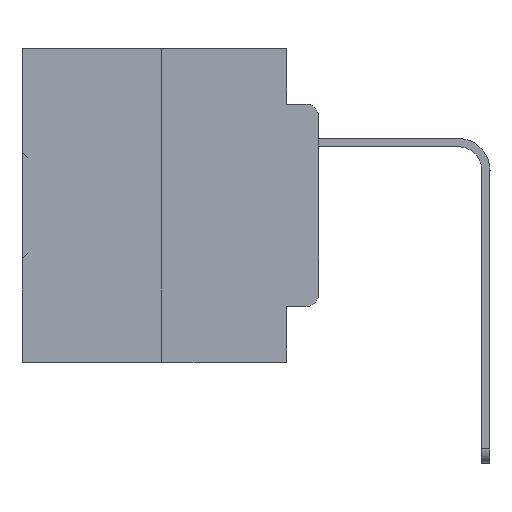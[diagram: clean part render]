
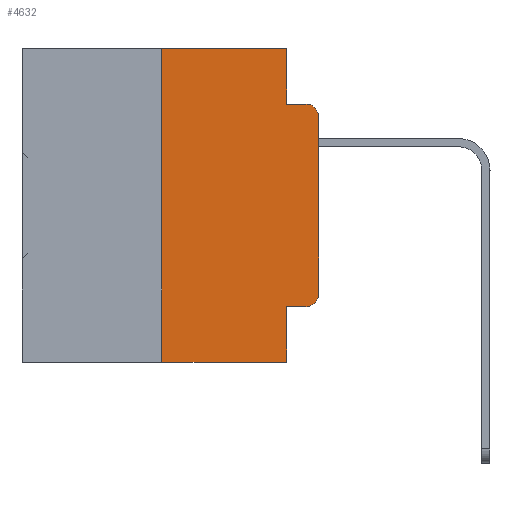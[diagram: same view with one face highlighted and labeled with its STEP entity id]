
A CAD part, left-side view. The second image highlights one B-rep face of the part: STEP entity #4632.
In plain terms, the highlighted planar face has unit normal (-1, 0, 0).
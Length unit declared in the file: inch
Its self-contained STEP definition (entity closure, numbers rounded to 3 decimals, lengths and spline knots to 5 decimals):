
#1252 = DIRECTION ( 'NONE',  ( 0., 0., -1. ) ) ;
#1343 = DIRECTION ( 'NONE',  ( 0., 0., -1. ) ) ;
#1459 = EDGE_CURVE ( 'NONE', #8099, #14613, #27639, .T. ) ;
#1803 = EDGE_CURVE ( 'NONE', #5049, #16139, #24611, .T. ) ;
#1824 = LINE ( 'NONE', #24914, #20456 ) ;
#1993 = LINE ( 'NONE', #28697, #35735 ) ;
#2382 = ORIENTED_EDGE ( 'NONE', *, *, #1803, .F. ) ;
#3555 = ORIENTED_EDGE ( 'NONE', *, *, #18162, .T. ) ;
#3873 = ORIENTED_EDGE ( 'NONE', *, *, #33376, .T. ) ;
#4410 = VERTEX_POINT ( 'NONE', #18798 ) ;
#4632 = ADVANCED_FACE ( 'NONE', ( #6417 ), #9212, .F. ) ;
#5018 = AXIS2_PLACEMENT_3D ( 'NONE', #8006, #21920, #16122 ) ;
#5049 = VERTEX_POINT ( 'NONE', #10887 ) ;
#5276 = CARTESIAN_POINT ( 'NONE',  ( 0., 0.473, -0.5 ) ) ;
#6052 = CARTESIAN_POINT ( 'NONE',  ( 0., 0.051, -0.5 ) ) ;
#6417 = FACE_OUTER_BOUND ( 'NONE', #10065, .T. ) ;
#6690 = ORIENTED_EDGE ( 'NONE', *, *, #1459, .T. ) ;
#7670 = ORIENTED_EDGE ( 'NONE', *, *, #20292, .F. ) ;
#8006 = CARTESIAN_POINT ( 'NONE',  ( 0., 0.02, -0.1085 ) ) ;
#8099 = VERTEX_POINT ( 'NONE', #27360 ) ;
#8934 = DIRECTION ( 'NONE',  ( 0., 0., -1. ) ) ;
#9212 = PLANE ( 'NONE',  #11813 ) ;
#9758 = ORIENTED_EDGE ( 'NONE', *, *, #31690, .F. ) ;
#10065 = EDGE_LOOP ( 'NONE', ( #6690, #16196, #12038, #7670, #9758, #2382, #22916, #22209, #3555, #3873 ) ) ;
#10873 = DIRECTION ( 'NONE',  ( 0., -1., 0. ) ) ;
#10887 = CARTESIAN_POINT ( 'NONE',  ( 0., 0.25, -0.5 ) ) ;
#10964 = CARTESIAN_POINT ( 'NONE',  ( 0., 0.051, 0. ) ) ;
#11242 = CARTESIAN_POINT ( 'NONE',  ( 0., 0.051, 0. ) ) ;
#11813 = AXIS2_PLACEMENT_3D ( 'NONE', #25563, #34114, #28425 ) ;
#12009 = VECTOR ( 'NONE', #32639, 39.37008 ) ;
#12038 = ORIENTED_EDGE ( 'NONE', *, *, #23349, .F. ) ;
#12192 = VECTOR ( 'NONE', #27050, 39.37008 ) ;
#13952 = AXIS2_PLACEMENT_3D ( 'NONE', #17846, #28818, #1252 ) ;
#14228 = VECTOR ( 'NONE', #30840, 39.37008 ) ;
#14613 = VERTEX_POINT ( 'NONE', #27564 ) ;
#14933 = DIRECTION ( 'NONE',  ( 0., -1., 0. ) ) ;
#15021 = LINE ( 'NONE', #32403, #12009 ) ;
#16122 = DIRECTION ( 'NONE',  ( 0., 0., -1. ) ) ;
#16139 = VERTEX_POINT ( 'NONE', #23440 ) ;
#16196 = ORIENTED_EDGE ( 'NONE', *, *, #31900, .T. ) ;
#17742 = EDGE_CURVE ( 'NONE', #4410, #28967, #23710, .T. ) ;
#17846 = CARTESIAN_POINT ( 'NONE',  ( 0., 0.02, -0.3915 ) ) ;
#18162 = EDGE_CURVE ( 'NONE', #4410, #25812, #15021, .T. ) ;
#18798 = CARTESIAN_POINT ( 'NONE',  ( 0., 0.051, -0.4115 ) ) ;
#18948 = CARTESIAN_POINT ( 'NONE',  ( 0., 0.25, 0. ) ) ;
#19159 = LINE ( 'NONE', #5276, #12192 ) ;
#20292 = EDGE_CURVE ( 'NONE', #34715, #29030, #20521, .T. ) ;
#20357 = CARTESIAN_POINT ( 'NONE',  ( 0., 0.051, 0. ) ) ;
#20456 = VECTOR ( 'NONE', #10873, 39.37008 ) ;
#20521 = LINE ( 'NONE', #20357, #23999 ) ;
#21477 = CIRCLE ( 'NONE', #5018, 0.02 ) ;
#21920 = DIRECTION ( 'NONE',  ( -1., 0., 0. ) ) ;
#22209 = ORIENTED_EDGE ( 'NONE', *, *, #17742, .F. ) ;
#22571 = CARTESIAN_POINT ( 'NONE',  ( 0., 0.02, -0.4115 ) ) ;
#22916 = ORIENTED_EDGE ( 'NONE', *, *, #23726, .T. ) ;
#23349 = EDGE_CURVE ( 'NONE', #29030, #28290, #1824, .T. ) ;
#23440 = CARTESIAN_POINT ( 'NONE',  ( 0., 0.25, 0. ) ) ;
#23710 = LINE ( 'NONE', #11242, #31501 ) ;
#23726 = EDGE_CURVE ( 'NONE', #5049, #28967, #19159, .T. ) ;
#23999 = VECTOR ( 'NONE', #1343, 39.37008 ) ;
#24611 = LINE ( 'NONE', #18948, #34104 ) ;
#24914 = CARTESIAN_POINT ( 'NONE',  ( 0., 0.051, -0.0885 ) ) ;
#25193 = CARTESIAN_POINT ( 'NONE',  ( 0., 0., 0. ) ) ;
#25563 = CARTESIAN_POINT ( 'NONE',  ( 0., 0.473, 0. ) ) ;
#25812 = VERTEX_POINT ( 'NONE', #22571 ) ;
#27050 = DIRECTION ( 'NONE',  ( 0., -1., 0. ) ) ;
#27360 = CARTESIAN_POINT ( 'NONE',  ( 0., 0., -0.3915 ) ) ;
#27564 = CARTESIAN_POINT ( 'NONE',  ( 0., 0., -0.1085 ) ) ;
#27639 = LINE ( 'NONE', #25193, #14228 ) ;
#27924 = CIRCLE ( 'NONE', #13952, 0.02 ) ;
#28290 = VERTEX_POINT ( 'NONE', #30309 ) ;
#28425 = DIRECTION ( 'NONE',  ( 0., 0., -1. ) ) ;
#28697 = CARTESIAN_POINT ( 'NONE',  ( 0., 0.473, 0. ) ) ;
#28818 = DIRECTION ( 'NONE',  ( -1., 0., 0. ) ) ;
#28967 = VERTEX_POINT ( 'NONE', #6052 ) ;
#29030 = VERTEX_POINT ( 'NONE', #30980 ) ;
#30309 = CARTESIAN_POINT ( 'NONE',  ( 0., 0.02, -0.0885 ) ) ;
#30840 = DIRECTION ( 'NONE',  ( 0., 0., 1. ) ) ;
#30980 = CARTESIAN_POINT ( 'NONE',  ( 0., 0.051, -0.0885 ) ) ;
#31501 = VECTOR ( 'NONE', #8934, 39.37008 ) ;
#31690 = EDGE_CURVE ( 'NONE', #16139, #34715, #1993, .T. ) ;
#31900 = EDGE_CURVE ( 'NONE', #14613, #28290, #21477, .T. ) ;
#32403 = CARTESIAN_POINT ( 'NONE',  ( 0., 0.051, -0.4115 ) ) ;
#32487 = DIRECTION ( 'NONE',  ( 0., 0., 1. ) ) ;
#32639 = DIRECTION ( 'NONE',  ( 0., -1., 0. ) ) ;
#33376 = EDGE_CURVE ( 'NONE', #25812, #8099, #27924, .T. ) ;
#34104 = VECTOR ( 'NONE', #32487, 39.37008 ) ;
#34114 = DIRECTION ( 'NONE',  ( 1., 0., 0. ) ) ;
#34715 = VERTEX_POINT ( 'NONE', #10964 ) ;
#35735 = VECTOR ( 'NONE', #14933, 39.37008 ) ;
